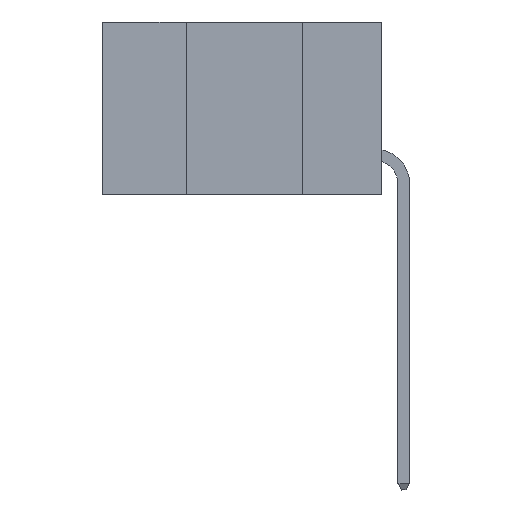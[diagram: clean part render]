
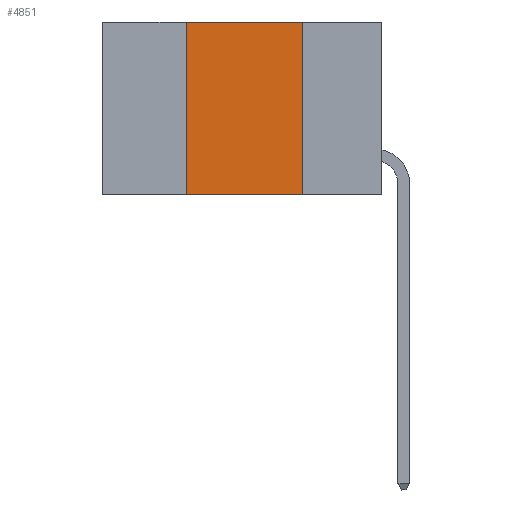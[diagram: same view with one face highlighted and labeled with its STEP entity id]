
A CAD part, left-side view. The second image highlights one B-rep face of the part: STEP entity #4851.
In plain terms, the highlighted planar face has unit normal (-1, 0, 0).
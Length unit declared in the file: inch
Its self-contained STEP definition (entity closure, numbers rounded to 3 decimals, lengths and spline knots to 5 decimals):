
#1112 = ORIENTED_EDGE ( 'NONE', *, *, #18051, .F. ) ;
#1675 = LINE ( 'NONE', #4965, #19147 ) ;
#2385 = EDGE_CURVE ( 'NONE', #9538, #20200, #15538, .T. ) ;
#2805 = CARTESIAN_POINT ( 'NONE',  ( 0., 0.17, 0. ) ) ;
#4573 = VECTOR ( 'NONE', #21421, 39.37008 ) ;
#4851 = ADVANCED_FACE ( 'NONE', ( #10868 ), #8198, .F. ) ;
#4965 = CARTESIAN_POINT ( 'NONE',  ( 0., 0.42, 0. ) ) ;
#5889 = DIRECTION ( 'NONE',  ( 0., -1., 0. ) ) ;
#6615 = CARTESIAN_POINT ( 'NONE',  ( 0., 0.17, 0. ) ) ;
#6854 = ORIENTED_EDGE ( 'NONE', *, *, #6912, .T. ) ;
#6912 = EDGE_CURVE ( 'NONE', #15832, #10815, #8547, .T. ) ;
#8198 = PLANE ( 'NONE',  #11573 ) ;
#8547 = LINE ( 'NONE', #17302, #13539 ) ;
#8656 = VECTOR ( 'NONE', #17782, 39.37008 ) ;
#9538 = VERTEX_POINT ( 'NONE', #18626 ) ;
#9975 = CARTESIAN_POINT ( 'NONE',  ( 0., 0.6, 0. ) ) ;
#10447 = EDGE_LOOP ( 'NONE', ( #12079, #21277, #1112, #6854 ) ) ;
#10815 = VERTEX_POINT ( 'NONE', #12703 ) ;
#10868 = FACE_OUTER_BOUND ( 'NONE', #10447, .T. ) ;
#11573 = AXIS2_PLACEMENT_3D ( 'NONE', #9975, #16556, #13102 ) ;
#12079 = ORIENTED_EDGE ( 'NONE', *, *, #13307, .F. ) ;
#12703 = CARTESIAN_POINT ( 'NONE',  ( 0., 0.17, -0.37 ) ) ;
#13102 = DIRECTION ( 'NONE',  ( 0., 0., -1. ) ) ;
#13307 = EDGE_CURVE ( 'NONE', #20200, #10815, #17792, .T. ) ;
#13468 = DIRECTION ( 'NONE',  ( 0., 0., 1. ) ) ;
#13539 = VECTOR ( 'NONE', #5889, 39.37008 ) ;
#15538 = LINE ( 'NONE', #16065, #8656 ) ;
#15832 = VERTEX_POINT ( 'NONE', #19584 ) ;
#16065 = CARTESIAN_POINT ( 'NONE',  ( 0., 0.6, 0. ) ) ;
#16556 = DIRECTION ( 'NONE',  ( 1., 0., 0. ) ) ;
#17302 = CARTESIAN_POINT ( 'NONE',  ( 0., 0.6, -0.37 ) ) ;
#17782 = DIRECTION ( 'NONE',  ( 0., -1., 0. ) ) ;
#17792 = LINE ( 'NONE', #2805, #4573 ) ;
#18051 = EDGE_CURVE ( 'NONE', #15832, #9538, #1675, .T. ) ;
#18626 = CARTESIAN_POINT ( 'NONE',  ( 0., 0.42, 0. ) ) ;
#19147 = VECTOR ( 'NONE', #13468, 39.37008 ) ;
#19584 = CARTESIAN_POINT ( 'NONE',  ( 0., 0.42, -0.37 ) ) ;
#20200 = VERTEX_POINT ( 'NONE', #6615 ) ;
#21277 = ORIENTED_EDGE ( 'NONE', *, *, #2385, .F. ) ;
#21421 = DIRECTION ( 'NONE',  ( 0., 0., -1. ) ) ;
